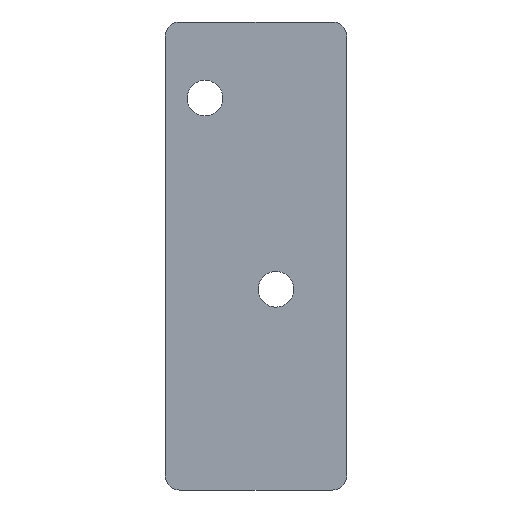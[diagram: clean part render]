
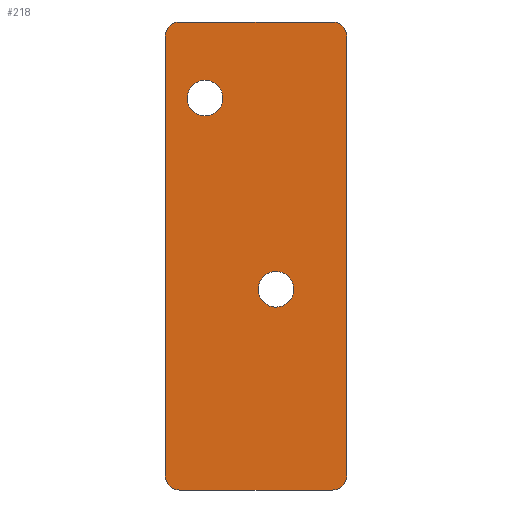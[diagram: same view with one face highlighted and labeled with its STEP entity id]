
A CAD part, left-side view. The second image highlights one B-rep face of the part: STEP entity #218.
In plain terms, the highlighted planar face has unit normal (-1, 0, 0).
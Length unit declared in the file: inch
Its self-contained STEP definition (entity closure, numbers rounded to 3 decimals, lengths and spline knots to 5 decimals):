
#15=FACE_BOUND('',#39,.T.);
#16=FACE_BOUND('',#40,.T.);
#19=PLANE('',#246);
#26=FACE_OUTER_BOUND('',#38,.T.);
#38=EDGE_LOOP('',(#155,#156,#157,#158,#159,#160,#161,#162));
#39=EDGE_LOOP('',(#163));
#40=EDGE_LOOP('',(#164));
#55=LINE('',#347,#73);
#56=LINE('',#351,#74);
#57=LINE('',#355,#75);
#58=LINE('',#358,#76);
#73=VECTOR('',#279,0.3937);
#74=VECTOR('',#282,0.3937);
#75=VECTOR('',#285,0.3937);
#76=VECTOR('',#288,0.3937);
#89=CIRCLE('',#244,0.0625);
#91=CIRCLE('',#247,0.0625);
#92=CIRCLE('',#248,0.0625);
#93=CIRCLE('',#249,0.0625);
#94=CIRCLE('',#250,0.07865);
#95=CIRCLE('',#251,0.07865);
#101=VERTEX_POINT('',#337);
#102=VERTEX_POINT('',#338);
#105=VERTEX_POINT('',#346);
#106=VERTEX_POINT('',#348);
#107=VERTEX_POINT('',#350);
#108=VERTEX_POINT('',#352);
#109=VERTEX_POINT('',#354);
#110=VERTEX_POINT('',#356);
#111=VERTEX_POINT('',#359);
#112=VERTEX_POINT('',#361);
#121=EDGE_CURVE('',#101,#102,#89,.T.);
#125=EDGE_CURVE('',#105,#101,#55,.T.);
#126=EDGE_CURVE('',#106,#105,#91,.T.);
#127=EDGE_CURVE('',#106,#107,#56,.T.);
#128=EDGE_CURVE('',#108,#107,#92,.T.);
#129=EDGE_CURVE('',#108,#109,#57,.T.);
#130=EDGE_CURVE('',#110,#109,#93,.T.);
#131=EDGE_CURVE('',#102,#110,#58,.F.);
#132=EDGE_CURVE('',#111,#111,#94,.T.);
#133=EDGE_CURVE('',#112,#112,#95,.T.);
#155=ORIENTED_EDGE('',*,*,#121,.F.);
#156=ORIENTED_EDGE('',*,*,#125,.F.);
#157=ORIENTED_EDGE('',*,*,#126,.F.);
#158=ORIENTED_EDGE('',*,*,#127,.T.);
#159=ORIENTED_EDGE('',*,*,#128,.F.);
#160=ORIENTED_EDGE('',*,*,#129,.T.);
#161=ORIENTED_EDGE('',*,*,#130,.F.);
#162=ORIENTED_EDGE('',*,*,#131,.F.);
#163=ORIENTED_EDGE('',*,*,#132,.T.);
#164=ORIENTED_EDGE('',*,*,#133,.T.);
#218=ADVANCED_FACE('',(#26,#15,#16),#19,.T.);
#244=AXIS2_PLACEMENT_3D('',#339,#271,#272);
#246=AXIS2_PLACEMENT_3D('',#345,#277,#278);
#247=AXIS2_PLACEMENT_3D('',#349,#280,#281);
#248=AXIS2_PLACEMENT_3D('',#353,#283,#284);
#249=AXIS2_PLACEMENT_3D('',#357,#286,#287);
#250=AXIS2_PLACEMENT_3D('',#360,#289,#290);
#251=AXIS2_PLACEMENT_3D('',#362,#291,#292);
#271=DIRECTION('center_axis',(1.,0.,0.));
#272=DIRECTION('ref_axis',(0.,-0.707,0.707));
#277=DIRECTION('center_axis',(-1.,0.,0.));
#278=DIRECTION('ref_axis',(0.,0.,-1.));
#279=DIRECTION('',(0.,-1.,0.));
#280=DIRECTION('center_axis',(1.,0.,0.));
#281=DIRECTION('ref_axis',(0.,0.707,0.707));
#282=DIRECTION('',(0.,0.,-1.));
#283=DIRECTION('center_axis',(1.,0.,0.));
#284=DIRECTION('ref_axis',(0.,0.707,-0.707));
#285=DIRECTION('',(0.,-1.,0.));
#286=DIRECTION('center_axis',(1.,0.,0.));
#287=DIRECTION('ref_axis',(0.,-0.707,-0.707));
#288=DIRECTION('',(0.,0.,1.));
#289=DIRECTION('center_axis',(1.,0.,0.));
#290=DIRECTION('ref_axis',(0.,0.,-1.));
#291=DIRECTION('center_axis',(1.,0.,0.));
#292=DIRECTION('ref_axis',(0.,0.,-1.));
#337=CARTESIAN_POINT('',(-0.363,-1.18756,-0.00394));
#338=CARTESIAN_POINT('',(-0.363,-1.25006,-0.06644));
#339=CARTESIAN_POINT('Origin',(-0.363,-1.18756,-0.06644));
#345=CARTESIAN_POINT('Origin',(-0.363,-0.45,0.));
#346=CARTESIAN_POINT('',(-0.363,-0.5125,-0.00394));
#347=CARTESIAN_POINT('',(-0.363,-0.45,-0.00394));
#348=CARTESIAN_POINT('',(-0.363,-0.45,-0.06644));
#349=CARTESIAN_POINT('Origin',(-0.363,-0.5125,-0.06644));
#350=CARTESIAN_POINT('',(-0.363,-0.45,-2.0075));
#351=CARTESIAN_POINT('',(-0.363,-0.45,-0.66275));
#352=CARTESIAN_POINT('',(-0.363,-0.5125,-2.07));
#353=CARTESIAN_POINT('Origin',(-0.363,-0.5125,-2.0075));
#354=CARTESIAN_POINT('',(-0.363,-1.18756,-2.07));
#355=CARTESIAN_POINT('',(-0.363,-0.45,-2.07));
#356=CARTESIAN_POINT('',(-0.363,-1.25006,-2.0075));
#357=CARTESIAN_POINT('Origin',(-0.363,-1.18756,-2.0075));
#358=CARTESIAN_POINT('',(-0.363,-1.25006,-0.66275));
#359=CARTESIAN_POINT('',(-0.363,-0.938,-1.10535));
#360=CARTESIAN_POINT('Origin',(-0.363,-0.938,-1.184));
#361=CARTESIAN_POINT('',(-0.363,-0.625,-0.26135));
#362=CARTESIAN_POINT('Origin',(-0.363,-0.625,-0.34));
